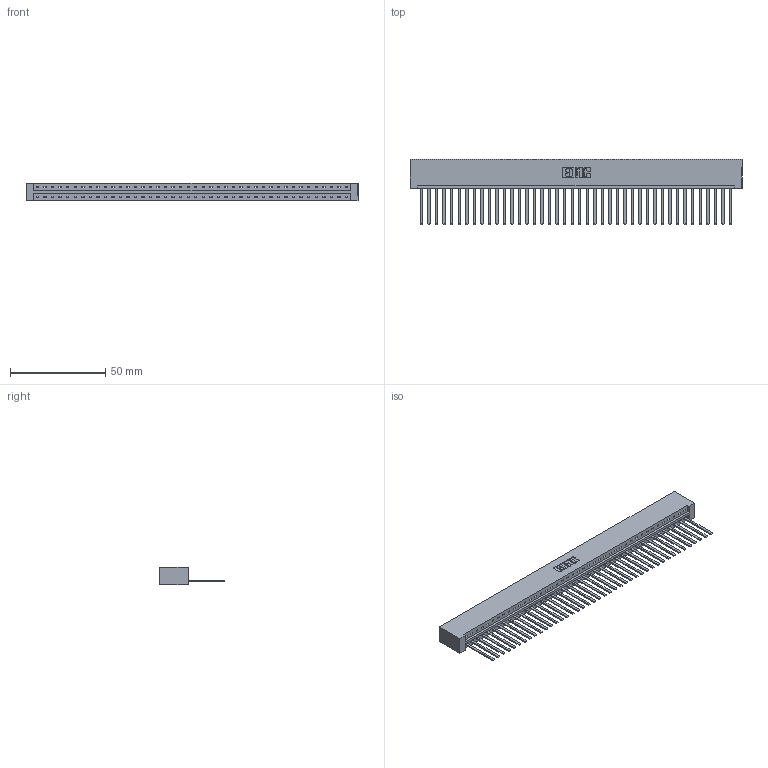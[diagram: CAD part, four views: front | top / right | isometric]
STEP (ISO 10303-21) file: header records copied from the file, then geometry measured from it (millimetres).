
FILE_DESCRIPTION (( 'STEP AP203' ), '1' );
FILE_NAME ('833-042-544-101.STEP', '2020-06-03T21:54:47', ( '' ), ( '' ), 'SwSTEP 2.0', 'SolidWorks 2020', '' );
FILE_SCHEMA (( 'CONFIG_CONTROL_DESIGN' ));
Length unit declared in the file: inch
Products named in the file (3): 345-292-001_345-293-144; 833 Part_Lugless; 833-042-544-101
Assembly tree (43 placements, depth 2):
  833-042-544-101
    833 Part_Lugless
    345-292-001_345-293-144  x42
Bounding box: 174.68 x 34.3 x 9.4 mm (x, y, z)
Volume: 18676.5 mm3; surface area: 21745.8 mm2
Topology: 43 solids, 43 shells, 2290 faces, 6923 edges, 4558 vertices
Faces by surface type: plane 1662, cylinder 628
Entity records: 25215 total; most frequent: CARTESIAN_POINT 4356, ORIENTED_EDGE 4334, DIRECTION 3663, EDGE_CURVE 2167, VECTOR 2051, LINE 2051, VERTEX_POINT 1442, AXIS2_PLACEMENT_3D 806
